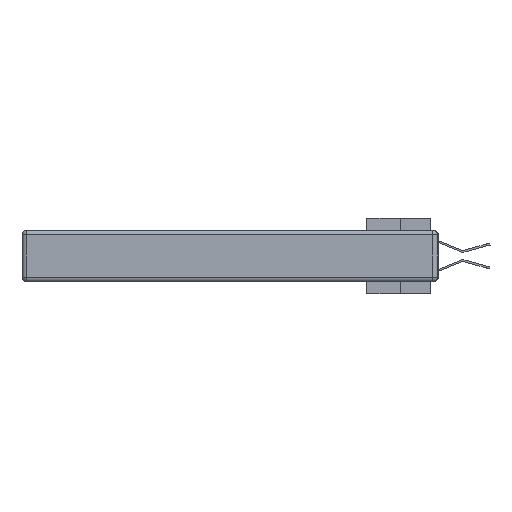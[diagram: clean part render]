
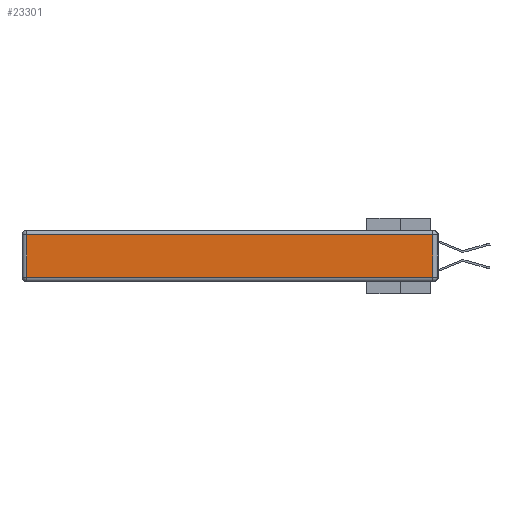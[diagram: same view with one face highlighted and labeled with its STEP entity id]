
A CAD part, left-side view. The second image highlights one B-rep face of the part: STEP entity #23301.
In plain terms, the highlighted planar face has unit normal (-1, 0, 0).
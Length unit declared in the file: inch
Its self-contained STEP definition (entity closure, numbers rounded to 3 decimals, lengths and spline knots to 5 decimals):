
#383 = VERTEX_POINT ( 'NONE', #27190 ) ;
#948 = EDGE_CURVE ( 'NONE', #5059, #2307, #5519, .T. ) ;
#1097 = CARTESIAN_POINT ( 'NONE',  ( 0., 0., -0.313 ) ) ;
#1139 = CARTESIAN_POINT ( 'NONE',  ( 0., 2.72, -0.313 ) ) ;
#1624 = LINE ( 'NONE', #15471, #29049 ) ;
#2307 = VERTEX_POINT ( 'NONE', #19268 ) ;
#2604 = ORIENTED_EDGE ( 'NONE', *, *, #948, .T. ) ;
#4038 = LINE ( 'NONE', #30242, #28177 ) ;
#4570 = LINE ( 'NONE', #1097, #28703 ) ;
#4780 = AXIS2_PLACEMENT_3D ( 'NONE', #21217, #28413, #14402 ) ;
#5059 = VERTEX_POINT ( 'NONE', #28790 ) ;
#5191 = EDGE_CURVE ( 'NONE', #2307, #383, #1624, .T. ) ;
#5519 = LINE ( 'NONE', #8009, #16513 ) ;
#7220 = VERTEX_POINT ( 'NONE', #1139 ) ;
#7309 = FACE_OUTER_BOUND ( 'NONE', #21322, .T. ) ;
#7389 = EDGE_CURVE ( 'NONE', #383, #7220, #4038, .T. ) ;
#8009 = CARTESIAN_POINT ( 'NONE',  ( 0., 0.03, -0.343 ) ) ;
#10054 = DIRECTION ( 'NONE',  ( 0., -1., 0. ) ) ;
#10805 = EDGE_CURVE ( 'NONE', #7220, #5059, #4570, .T. ) ;
#14402 = DIRECTION ( 'NONE',  ( 0., 0., 1. ) ) ;
#15471 = CARTESIAN_POINT ( 'NONE',  ( 0., 2.75, -0.03 ) ) ;
#16513 = VECTOR ( 'NONE', #24387, 39.37008 ) ;
#16553 = ORIENTED_EDGE ( 'NONE', *, *, #7389, .T. ) ;
#19268 = CARTESIAN_POINT ( 'NONE',  ( 0., 0.03, -0.03 ) ) ;
#20539 = DIRECTION ( 'NONE',  ( 0., 0., -1. ) ) ;
#21217 = CARTESIAN_POINT ( 'NONE',  ( 0., 0., -0.343 ) ) ;
#21322 = EDGE_LOOP ( 'NONE', ( #26962, #2604, #22102, #16553 ) ) ;
#22102 = ORIENTED_EDGE ( 'NONE', *, *, #5191, .T. ) ;
#23301 = ADVANCED_FACE ( 'NONE', ( #7309 ), #23747, .T. ) ;
#23747 = PLANE ( 'NONE',  #4780 ) ;
#24387 = DIRECTION ( 'NONE',  ( 0., 0., 1. ) ) ;
#26962 = ORIENTED_EDGE ( 'NONE', *, *, #10805, .T. ) ;
#27029 = DIRECTION ( 'NONE',  ( 0., 1., 0. ) ) ;
#27190 = CARTESIAN_POINT ( 'NONE',  ( 0., 2.72, -0.03 ) ) ;
#28177 = VECTOR ( 'NONE', #20539, 39.37008 ) ;
#28413 = DIRECTION ( 'NONE',  ( -1., 0., 0. ) ) ;
#28703 = VECTOR ( 'NONE', #10054, 39.37008 ) ;
#28790 = CARTESIAN_POINT ( 'NONE',  ( 0., 0.03, -0.313 ) ) ;
#29049 = VECTOR ( 'NONE', #27029, 39.37008 ) ;
#30242 = CARTESIAN_POINT ( 'NONE',  ( 0., 2.72, -0.343 ) ) ;
